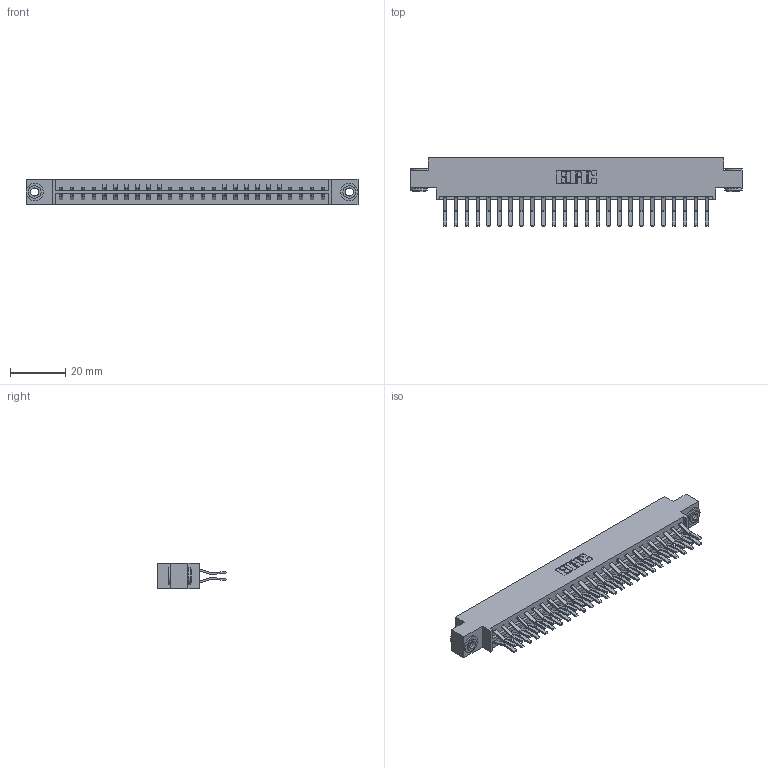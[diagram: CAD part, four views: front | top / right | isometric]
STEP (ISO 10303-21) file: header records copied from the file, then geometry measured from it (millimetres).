
FILE_DESCRIPTION (( 'STEP AP203' ), '1' );
FILE_NAME ('833-050-560-803.STEP', '2020-06-04T18:29:09', ( '' ), ( '' ), 'SwSTEP 2.0', 'SolidWorks 2020', '' );
FILE_SCHEMA (( 'CONFIG_CONTROL_DESIGN' ));
Length unit declared in the file: inch
Products named in the file (4): 345-292-001_560 Tail; 833 Part_Offset - .156 Dia - TH; 833-050-560-803; 345-250-002_345-250-002-102
Assembly tree (53 placements, depth 2):
  833-050-560-803
    833 Part_Offset - .156 Dia - TH
    345-292-001_560 Tail  x50
    345-250-002_345-250-002-102  x2
Bounding box: 120.6 x 24.78 x 9.4 mm (x, y, z)
Volume: 12272.8 mm3; surface area: 15703.5 mm2
Topology: 53 solids, 53 shells, 2856 faces, 8449 edges, 5562 vertices
Faces by surface type: plane 1884, cylinder 964, cone 8
Entity records: 19152 total; most frequent: CARTESIAN_POINT 3173, ORIENTED_EDGE 3102, DIRECTION 2777, EDGE_CURVE 1551, VECTOR 1395, LINE 1395, VERTEX_POINT 1030, AXIS2_PLACEMENT_3D 691
